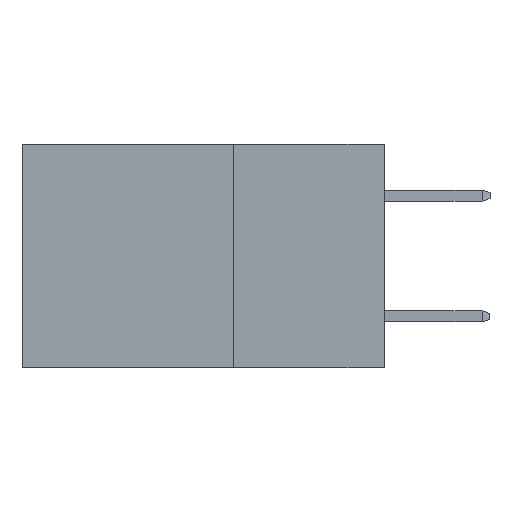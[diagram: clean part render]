
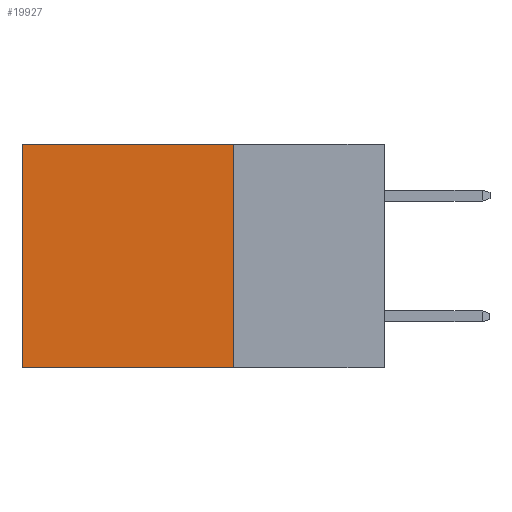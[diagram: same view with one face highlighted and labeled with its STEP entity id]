
A CAD part, left-side view. The second image highlights one B-rep face of the part: STEP entity #19927.
In plain terms, the highlighted planar face has unit normal (-1, 0, 0).
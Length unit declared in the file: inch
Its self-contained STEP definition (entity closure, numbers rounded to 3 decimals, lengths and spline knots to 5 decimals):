
#1416 = LINE ( 'NONE', #2433, #23942 ) ;
#1856 = ORIENTED_EDGE ( 'NONE', *, *, #21477, .T. ) ;
#2181 = FACE_OUTER_BOUND ( 'NONE', #5702, .T. ) ;
#2421 = DIRECTION ( 'NONE',  ( 0., 0., -1. ) ) ;
#2433 = CARTESIAN_POINT ( 'NONE',  ( 0.298, 0.25, -0.37 ) ) ;
#2521 = VERTEX_POINT ( 'NONE', #17655 ) ;
#3042 = LINE ( 'NONE', #21517, #19317 ) ;
#4246 = EDGE_CURVE ( 'NONE', #2521, #16805, #1416, .T. ) ;
#4343 = CARTESIAN_POINT ( 'NONE',  ( 0.298, 0.25, 0. ) ) ;
#5702 = EDGE_LOOP ( 'NONE', ( #1856, #19904, #7458, #12066 ) ) ;
#6756 = CARTESIAN_POINT ( 'NONE',  ( 0.298, 0.6, 0. ) ) ;
#6944 = CARTESIAN_POINT ( 'NONE',  ( 0.298, 0.25, 0. ) ) ;
#7458 = ORIENTED_EDGE ( 'NONE', *, *, #16179, .F. ) ;
#8725 = VECTOR ( 'NONE', #18712, 39.37008 ) ;
#9108 = DIRECTION ( 'NONE',  ( 0., 0., -1. ) ) ;
#10730 = DIRECTION ( 'NONE',  ( 0., 1., 0. ) ) ;
#10839 = CARTESIAN_POINT ( 'NONE',  ( 0.298, 0.6, -0.37 ) ) ;
#11415 = AXIS2_PLACEMENT_3D ( 'NONE', #6944, #21734, #9108 ) ;
#11937 = LINE ( 'NONE', #4343, #22431 ) ;
#12066 = ORIENTED_EDGE ( 'NONE', *, *, #19784, .T. ) ;
#13744 = VERTEX_POINT ( 'NONE', #14930 ) ;
#14930 = CARTESIAN_POINT ( 'NONE',  ( 0.298, 0.25, 0. ) ) ;
#16179 = EDGE_CURVE ( 'NONE', #13744, #2521, #3042, .T. ) ;
#16601 = CARTESIAN_POINT ( 'NONE',  ( 0.298, 0.6, 0. ) ) ;
#16805 = VERTEX_POINT ( 'NONE', #10839 ) ;
#17655 = CARTESIAN_POINT ( 'NONE',  ( 0.298, 0.25, -0.37 ) ) ;
#18712 = DIRECTION ( 'NONE',  ( 0., 0., -1. ) ) ;
#19317 = VECTOR ( 'NONE', #2421, 39.37008 ) ;
#19645 = PLANE ( 'NONE',  #11415 ) ;
#19784 = EDGE_CURVE ( 'NONE', #13744, #23171, #11937, .T. ) ;
#19904 = ORIENTED_EDGE ( 'NONE', *, *, #4246, .F. ) ;
#19927 = ADVANCED_FACE ( 'NONE', ( #2181 ), #19645, .F. ) ;
#21477 = EDGE_CURVE ( 'NONE', #23171, #16805, #26144, .T. ) ;
#21517 = CARTESIAN_POINT ( 'NONE',  ( 0.298, 0.25, 0. ) ) ;
#21734 = DIRECTION ( 'NONE',  ( 1., 0., 0. ) ) ;
#22431 = VECTOR ( 'NONE', #10730, 39.37008 ) ;
#23171 = VERTEX_POINT ( 'NONE', #6756 ) ;
#23942 = VECTOR ( 'NONE', #25638, 39.37008 ) ;
#25638 = DIRECTION ( 'NONE',  ( 0., 1., 0. ) ) ;
#26144 = LINE ( 'NONE', #16601, #8725 ) ;
